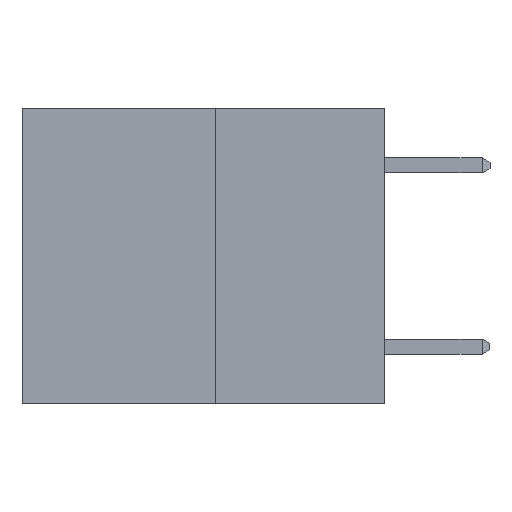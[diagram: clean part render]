
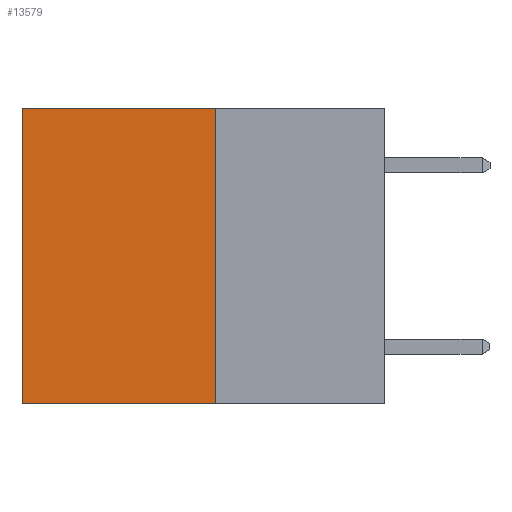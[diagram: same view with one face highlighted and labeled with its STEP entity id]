
A CAD part, left-side view. The second image highlights one B-rep face of the part: STEP entity #13579.
In plain terms, the highlighted planar face has unit normal (-1, 0, 0).
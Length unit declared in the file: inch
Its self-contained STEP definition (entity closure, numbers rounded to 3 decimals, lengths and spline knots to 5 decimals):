
#221 = CARTESIAN_POINT ( 'NONE',  ( 0.3165, 0.28, -0.49 ) ) ;
#318 = EDGE_CURVE ( 'NONE', #13510, #9413, #13363, .T. ) ;
#2344 = PLANE ( 'NONE',  #14674 ) ;
#2911 = VECTOR ( 'NONE', #10958, 39.37008 ) ;
#3091 = CARTESIAN_POINT ( 'NONE',  ( 0.3165, 0.6, -0.49 ) ) ;
#3537 = EDGE_CURVE ( 'NONE', #17139, #4524, #8393, .T. ) ;
#4408 = EDGE_LOOP ( 'NONE', ( #16340, #6359, #13433, #13903 ) ) ;
#4524 = VERTEX_POINT ( 'NONE', #5990 ) ;
#5450 = DIRECTION ( 'NONE',  ( 1., 0., 0. ) ) ;
#5787 = LINE ( 'NONE', #17259, #2911 ) ;
#5990 = CARTESIAN_POINT ( 'NONE',  ( 0.3165, 0.28, -0.49 ) ) ;
#6359 = ORIENTED_EDGE ( 'NONE', *, *, #8412, .F. ) ;
#6539 = EDGE_CURVE ( 'NONE', #17139, #13510, #14733, .T. ) ;
#6624 = VECTOR ( 'NONE', #13877, 39.37008 ) ;
#7007 = DIRECTION ( 'NONE',  ( 0., 0., -1. ) ) ;
#8393 = LINE ( 'NONE', #221, #11303 ) ;
#8412 = EDGE_CURVE ( 'NONE', #4524, #9413, #5787, .T. ) ;
#9413 = VERTEX_POINT ( 'NONE', #9859 ) ;
#9859 = CARTESIAN_POINT ( 'NONE',  ( 0.3165, 0.6, -0.49 ) ) ;
#10824 = DIRECTION ( 'NONE',  ( 0., 0., -1. ) ) ;
#10843 = CARTESIAN_POINT ( 'NONE',  ( 0.3165, 0.28, 0. ) ) ;
#10958 = DIRECTION ( 'NONE',  ( 0., 1., 0. ) ) ;
#11050 = DIRECTION ( 'NONE',  ( 0., 1., 0. ) ) ;
#11269 = CARTESIAN_POINT ( 'NONE',  ( 0.3165, 0.28, 0. ) ) ;
#11303 = VECTOR ( 'NONE', #10824, 39.37008 ) ;
#13363 = LINE ( 'NONE', #3091, #6624 ) ;
#13433 = ORIENTED_EDGE ( 'NONE', *, *, #3537, .F. ) ;
#13510 = VERTEX_POINT ( 'NONE', #19195 ) ;
#13579 = ADVANCED_FACE ( 'NONE', ( #14589 ), #2344, .F. ) ;
#13758 = VECTOR ( 'NONE', #11050, 39.37008 ) ;
#13877 = DIRECTION ( 'NONE',  ( 0., 0., -1. ) ) ;
#13903 = ORIENTED_EDGE ( 'NONE', *, *, #6539, .T. ) ;
#14589 = FACE_OUTER_BOUND ( 'NONE', #4408, .T. ) ;
#14674 = AXIS2_PLACEMENT_3D ( 'NONE', #16312, #5450, #7007 ) ;
#14733 = LINE ( 'NONE', #10843, #13758 ) ;
#16312 = CARTESIAN_POINT ( 'NONE',  ( 0.3165, 0.28, -0.49 ) ) ;
#16340 = ORIENTED_EDGE ( 'NONE', *, *, #318, .T. ) ;
#17139 = VERTEX_POINT ( 'NONE', #11269 ) ;
#17259 = CARTESIAN_POINT ( 'NONE',  ( 0.3165, 0.28, -0.49 ) ) ;
#19195 = CARTESIAN_POINT ( 'NONE',  ( 0.3165, 0.6, 0. ) ) ;
